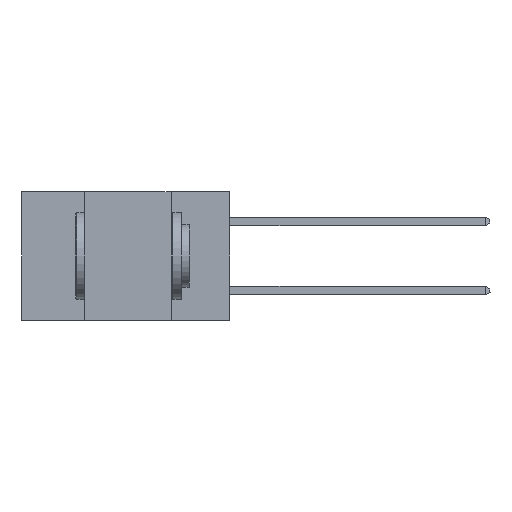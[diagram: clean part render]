
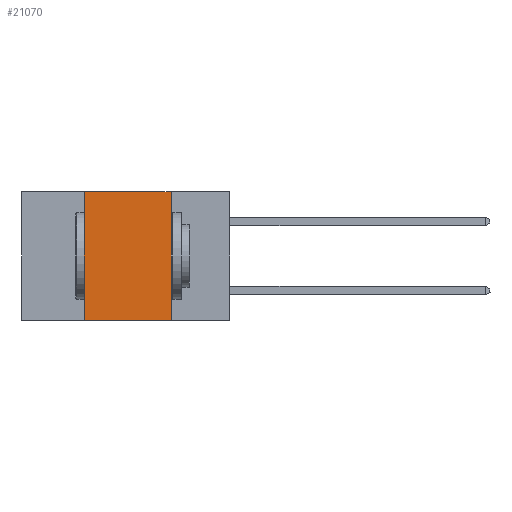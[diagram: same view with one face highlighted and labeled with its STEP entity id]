
A CAD part, left-side view. The second image highlights one B-rep face of the part: STEP entity #21070.
In plain terms, the highlighted planar face has unit normal (-1, 0, 0).
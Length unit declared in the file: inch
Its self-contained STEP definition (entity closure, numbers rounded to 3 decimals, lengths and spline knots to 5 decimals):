
#417 = VECTOR ( 'NONE', #15433, 39.37008 ) ;
#1451 = ORIENTED_EDGE ( 'NONE', *, *, #3434, .F. ) ;
#3434 = EDGE_CURVE ( 'NONE', #14098, #8238, #20062, .T. ) ;
#3514 = EDGE_CURVE ( 'NONE', #31703, #8238, #31625, .T. ) ;
#4248 = EDGE_CURVE ( 'NONE', #23042, #14098, #10368, .T. ) ;
#5653 = FACE_OUTER_BOUND ( 'NONE', #7046, .T. ) ;
#6036 = CARTESIAN_POINT ( 'NONE',  ( 0., 0.17, -0.37 ) ) ;
#6652 = DIRECTION ( 'NONE',  ( 0., 0., -1. ) ) ;
#6748 = AXIS2_PLACEMENT_3D ( 'NONE', #26717, #13868, #6652 ) ;
#7046 = EDGE_LOOP ( 'NONE', ( #1451, #27843, #18179, #29365 ) ) ;
#7723 = DIRECTION ( 'NONE',  ( 0., -1., 0. ) ) ;
#8238 = VERTEX_POINT ( 'NONE', #6036 ) ;
#8866 = EDGE_CURVE ( 'NONE', #31703, #23042, #9677, .T. ) ;
#9616 = VECTOR ( 'NONE', #16990, 39.37008 ) ;
#9677 = LINE ( 'NONE', #16910, #25111 ) ;
#10368 = LINE ( 'NONE', #29492, #9616 ) ;
#10405 = CARTESIAN_POINT ( 'NONE',  ( 0., 0.42, 0. ) ) ;
#11722 = PLANE ( 'NONE',  #6748 ) ;
#11878 = CARTESIAN_POINT ( 'NONE',  ( 0., 0.17, 0. ) ) ;
#11978 = CARTESIAN_POINT ( 'NONE',  ( 0., 0.42, -0.37 ) ) ;
#13868 = DIRECTION ( 'NONE',  ( 1., 0., 0. ) ) ;
#14098 = VERTEX_POINT ( 'NONE', #30508 ) ;
#14221 = DIRECTION ( 'NONE',  ( 0., 0., 1. ) ) ;
#15433 = DIRECTION ( 'NONE',  ( 0., 0., -1. ) ) ;
#16910 = CARTESIAN_POINT ( 'NONE',  ( 0., 0.42, 0. ) ) ;
#16990 = DIRECTION ( 'NONE',  ( 0., -1., 0. ) ) ;
#17349 = VECTOR ( 'NONE', #7723, 39.37008 ) ;
#18179 = ORIENTED_EDGE ( 'NONE', *, *, #8866, .F. ) ;
#20062 = LINE ( 'NONE', #11878, #417 ) ;
#21070 = ADVANCED_FACE ( 'NONE', ( #5653 ), #11722, .F. ) ;
#23042 = VERTEX_POINT ( 'NONE', #10405 ) ;
#25111 = VECTOR ( 'NONE', #14221, 39.37008 ) ;
#26717 = CARTESIAN_POINT ( 'NONE',  ( 0., 0.6, 0. ) ) ;
#27337 = CARTESIAN_POINT ( 'NONE',  ( 0., 0.6, -0.37 ) ) ;
#27843 = ORIENTED_EDGE ( 'NONE', *, *, #4248, .F. ) ;
#29365 = ORIENTED_EDGE ( 'NONE', *, *, #3514, .T. ) ;
#29492 = CARTESIAN_POINT ( 'NONE',  ( 0., 0.6, 0. ) ) ;
#30508 = CARTESIAN_POINT ( 'NONE',  ( 0., 0.17, 0. ) ) ;
#31625 = LINE ( 'NONE', #27337, #17349 ) ;
#31703 = VERTEX_POINT ( 'NONE', #11978 ) ;
